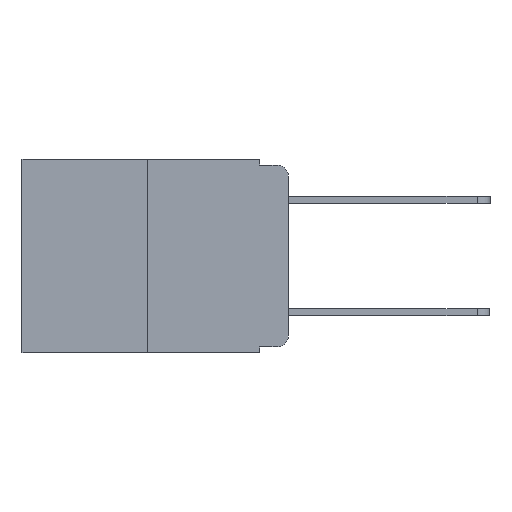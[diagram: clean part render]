
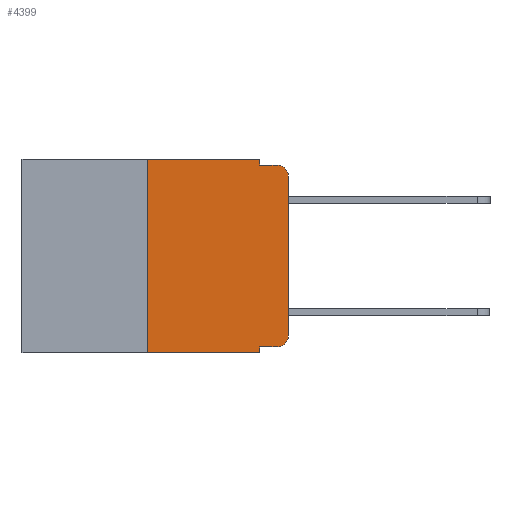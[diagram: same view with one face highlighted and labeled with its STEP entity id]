
A CAD part, left-side view. The second image highlights one B-rep face of the part: STEP entity #4399.
In plain terms, the highlighted planar face has unit normal (-1, 0, 0).
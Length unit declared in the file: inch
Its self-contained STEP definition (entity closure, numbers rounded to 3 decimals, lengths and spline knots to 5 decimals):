
#98 = DIRECTION ( 'NONE',  ( 0., 0., -1. ) ) ;
#395 = DIRECTION ( 'NONE',  ( 1., 0., 0. ) ) ;
#419 = VERTEX_POINT ( 'NONE', #3389 ) ;
#823 = AXIS2_PLACEMENT_3D ( 'NONE', #6180, #395, #12953 ) ;
#1256 = VERTEX_POINT ( 'NONE', #20715 ) ;
#1499 = EDGE_CURVE ( 'NONE', #419, #2678, #5777, .T. ) ;
#2453 = CARTESIAN_POINT ( 'NONE',  ( 0., 0.02, -0.03 ) ) ;
#2457 = VERTEX_POINT ( 'NONE', #9026 ) ;
#2554 = LINE ( 'NONE', #12130, #11467 ) ;
#2678 = VERTEX_POINT ( 'NONE', #17791 ) ;
#2795 = EDGE_CURVE ( 'NONE', #13174, #8477, #13352, .T. ) ;
#3361 = DIRECTION ( 'NONE',  ( 0., 0., -1. ) ) ;
#3389 = CARTESIAN_POINT ( 'NONE',  ( 0., 0.051, -0.333 ) ) ;
#4098 = EDGE_CURVE ( 'NONE', #1256, #16582, #15277, .T. ) ;
#4381 = DIRECTION ( 'NONE',  ( 0., 0., -1. ) ) ;
#4399 = ADVANCED_FACE ( 'NONE', ( #11505 ), #7932, .F. ) ;
#4439 = CARTESIAN_POINT ( 'NONE',  ( 0., 0.051, -0.01 ) ) ;
#4515 = ORIENTED_EDGE ( 'NONE', *, *, #18969, .T. ) ;
#4685 = CARTESIAN_POINT ( 'NONE',  ( 0., 0., -0.313 ) ) ;
#4990 = DIRECTION ( 'NONE',  ( 0., 0., -1. ) ) ;
#5012 = CARTESIAN_POINT ( 'NONE',  ( 0., 0., 0. ) ) ;
#5098 = ORIENTED_EDGE ( 'NONE', *, *, #15218, .F. ) ;
#5224 = CARTESIAN_POINT ( 'NONE',  ( 0., 0.02, -0.01 ) ) ;
#5777 = LINE ( 'NONE', #16914, #14173 ) ;
#6180 = CARTESIAN_POINT ( 'NONE',  ( 0., 0.473, 0. ) ) ;
#6244 = ORIENTED_EDGE ( 'NONE', *, *, #2795, .F. ) ;
#6565 = EDGE_CURVE ( 'NONE', #16582, #13743, #13388, .T. ) ;
#7339 = CIRCLE ( 'NONE', #15689, 0.02 ) ;
#7405 = EDGE_LOOP ( 'NONE', ( #21823, #13997, #21657, #10036, #5098, #6244, #13852, #18037, #8739, #4515 ) ) ;
#7745 = EDGE_CURVE ( 'NONE', #10703, #13743, #7339, .T. ) ;
#7932 = PLANE ( 'NONE',  #823 ) ;
#8312 = CARTESIAN_POINT ( 'NONE',  ( 0., 0.051, -0.01 ) ) ;
#8477 = VERTEX_POINT ( 'NONE', #8523 ) ;
#8523 = CARTESIAN_POINT ( 'NONE',  ( 0., 0.25, 0. ) ) ;
#8739 = ORIENTED_EDGE ( 'NONE', *, *, #21062, .T. ) ;
#9026 = CARTESIAN_POINT ( 'NONE',  ( 0., 0.02, -0.333 ) ) ;
#10036 = ORIENTED_EDGE ( 'NONE', *, *, #4098, .F. ) ;
#10548 = CIRCLE ( 'NONE', #12932, 0.02 ) ;
#10703 = VERTEX_POINT ( 'NONE', #13176 ) ;
#11145 = DIRECTION ( 'NONE',  ( -1., 0., 0. ) ) ;
#11467 = VECTOR ( 'NONE', #16400, 39.37008 ) ;
#11505 = FACE_OUTER_BOUND ( 'NONE', #7405, .T. ) ;
#11619 = VERTEX_POINT ( 'NONE', #4685 ) ;
#11858 = LINE ( 'NONE', #21214, #19753 ) ;
#11959 = DIRECTION ( 'NONE',  ( 0., 0., 1. ) ) ;
#12130 = CARTESIAN_POINT ( 'NONE',  ( 0., 0.051, -0.333 ) ) ;
#12256 = EDGE_CURVE ( 'NONE', #11619, #10703, #17321, .T. ) ;
#12610 = VECTOR ( 'NONE', #16685, 39.37008 ) ;
#12932 = AXIS2_PLACEMENT_3D ( 'NONE', #20573, #11145, #98 ) ;
#12953 = DIRECTION ( 'NONE',  ( 0., 0., -1. ) ) ;
#12995 = DIRECTION ( 'NONE',  ( 0., -1., 0. ) ) ;
#13174 = VERTEX_POINT ( 'NONE', #15282 ) ;
#13176 = CARTESIAN_POINT ( 'NONE',  ( 0., 0., -0.03 ) ) ;
#13352 = LINE ( 'NONE', #21377, #17564 ) ;
#13388 = LINE ( 'NONE', #4439, #21722 ) ;
#13743 = VERTEX_POINT ( 'NONE', #5224 ) ;
#13852 = ORIENTED_EDGE ( 'NONE', *, *, #16394, .T. ) ;
#13997 = ORIENTED_EDGE ( 'NONE', *, *, #7745, .T. ) ;
#14173 = VECTOR ( 'NONE', #3361, 39.37008 ) ;
#14553 = DIRECTION ( 'NONE',  ( -1., 0., 0. ) ) ;
#15218 = EDGE_CURVE ( 'NONE', #8477, #1256, #11858, .T. ) ;
#15277 = LINE ( 'NONE', #16669, #20398 ) ;
#15282 = CARTESIAN_POINT ( 'NONE',  ( 0., 0.25, -0.343 ) ) ;
#15689 = AXIS2_PLACEMENT_3D ( 'NONE', #2453, #14553, #4381 ) ;
#15691 = DIRECTION ( 'NONE',  ( 0., -1., 0. ) ) ;
#16394 = EDGE_CURVE ( 'NONE', #13174, #2678, #21411, .T. ) ;
#16400 = DIRECTION ( 'NONE',  ( 0., -1., 0. ) ) ;
#16582 = VERTEX_POINT ( 'NONE', #8312 ) ;
#16669 = CARTESIAN_POINT ( 'NONE',  ( 0., 0.051, 0. ) ) ;
#16685 = DIRECTION ( 'NONE',  ( 0., 0., 1. ) ) ;
#16914 = CARTESIAN_POINT ( 'NONE',  ( 0., 0.051, 0. ) ) ;
#17294 = VECTOR ( 'NONE', #15691, 39.37008 ) ;
#17321 = LINE ( 'NONE', #5012, #12610 ) ;
#17564 = VECTOR ( 'NONE', #11959, 39.37008 ) ;
#17791 = CARTESIAN_POINT ( 'NONE',  ( 0., 0.051, -0.343 ) ) ;
#18037 = ORIENTED_EDGE ( 'NONE', *, *, #1499, .F. ) ;
#18969 = EDGE_CURVE ( 'NONE', #2457, #11619, #10548, .T. ) ;
#19647 = DIRECTION ( 'NONE',  ( 0., -1., 0. ) ) ;
#19753 = VECTOR ( 'NONE', #19647, 39.37008 ) ;
#20311 = CARTESIAN_POINT ( 'NONE',  ( 0., 0.473, -0.343 ) ) ;
#20398 = VECTOR ( 'NONE', #4990, 39.37008 ) ;
#20573 = CARTESIAN_POINT ( 'NONE',  ( 0., 0.02, -0.313 ) ) ;
#20715 = CARTESIAN_POINT ( 'NONE',  ( 0., 0.051, 0. ) ) ;
#21062 = EDGE_CURVE ( 'NONE', #419, #2457, #2554, .T. ) ;
#21214 = CARTESIAN_POINT ( 'NONE',  ( 0., 0.473, 0. ) ) ;
#21377 = CARTESIAN_POINT ( 'NONE',  ( 0., 0.25, 0. ) ) ;
#21411 = LINE ( 'NONE', #20311, #17294 ) ;
#21657 = ORIENTED_EDGE ( 'NONE', *, *, #6565, .F. ) ;
#21722 = VECTOR ( 'NONE', #12995, 39.37008 ) ;
#21823 = ORIENTED_EDGE ( 'NONE', *, *, #12256, .T. ) ;
